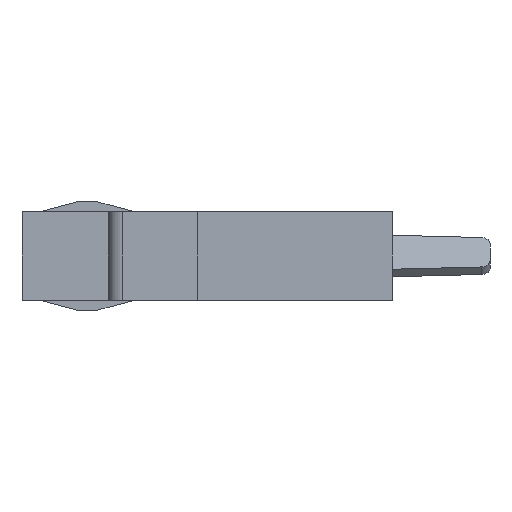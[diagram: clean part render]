
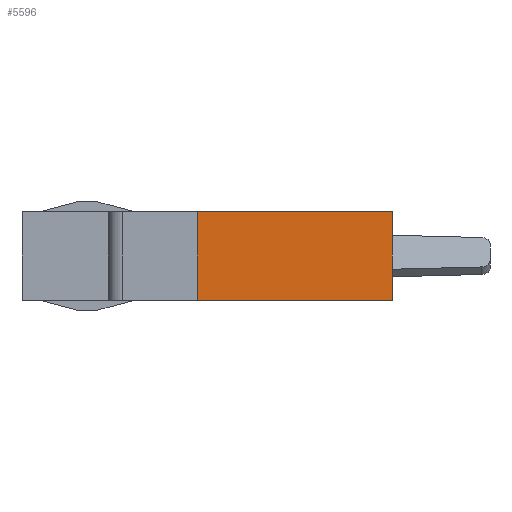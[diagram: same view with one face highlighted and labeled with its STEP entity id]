
A CAD part, left-side view. The second image highlights one B-rep face of the part: STEP entity #5596.
In plain terms, the highlighted planar face has unit normal (-1, 0, 0).
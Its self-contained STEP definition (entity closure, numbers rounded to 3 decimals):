
#51 = CARTESIAN_POINT ( 'NONE',  ( -2.235, 0., 2.54 ) ) ;
#229 = EDGE_CURVE ( 'NONE', #5375, #2570, #3643, .T. ) ;
#600 = CARTESIAN_POINT ( 'NONE',  ( -2.235, -11.176, -2.54 ) ) ;
#729 = LINE ( 'NONE', #5185, #3225 ) ;
#948 = CARTESIAN_POINT ( 'NONE',  ( -2.235, 0., 2.54 ) ) ;
#1081 = PLANE ( 'NONE',  #2968 ) ;
#1299 = LINE ( 'NONE', #3703, #6645 ) ;
#1427 = ORIENTED_EDGE ( 'NONE', *, *, #5101, .F. ) ;
#1739 = EDGE_CURVE ( 'NONE', #3036, #5375, #729, .T. ) ;
#2226 = DIRECTION ( 'NONE',  ( 0., 1., 0. ) ) ;
#2310 = LINE ( 'NONE', #948, #5884 ) ;
#2388 = DIRECTION ( 'NONE',  ( 0., 1., 0. ) ) ;
#2570 = VERTEX_POINT ( 'NONE', #51 ) ;
#2621 = DIRECTION ( 'NONE',  ( 0., 0., 1. ) ) ;
#2668 = DIRECTION ( 'NONE',  ( -1., 0., 0. ) ) ;
#2684 = ORIENTED_EDGE ( 'NONE', *, *, #1739, .T. ) ;
#2890 = CARTESIAN_POINT ( 'NONE',  ( -2.235, -11.176, 2.54 ) ) ;
#2968 = AXIS2_PLACEMENT_3D ( 'NONE', #600, #2668, #2621 ) ;
#3036 = VERTEX_POINT ( 'NONE', #5027 ) ;
#3225 = VECTOR ( 'NONE', #5701, 1000. ) ;
#3454 = VERTEX_POINT ( 'NONE', #4901 ) ;
#3611 = FACE_OUTER_BOUND ( 'NONE', #5616, .T. ) ;
#3643 = LINE ( 'NONE', #2890, #6347 ) ;
#3703 = CARTESIAN_POINT ( 'NONE',  ( -2.235, -11.176, -2.54 ) ) ;
#4626 = ORIENTED_EDGE ( 'NONE', *, *, #6004, .T. ) ;
#4901 = CARTESIAN_POINT ( 'NONE',  ( -2.235, 0., -2.54 ) ) ;
#4905 = ORIENTED_EDGE ( 'NONE', *, *, #229, .T. ) ;
#4911 = CARTESIAN_POINT ( 'NONE',  ( -2.235, -11.176, 2.54 ) ) ;
#5027 = CARTESIAN_POINT ( 'NONE',  ( -2.235, -11.176, -2.54 ) ) ;
#5101 = EDGE_CURVE ( 'NONE', #3036, #3454, #1299, .T. ) ;
#5185 = CARTESIAN_POINT ( 'NONE',  ( -2.235, -11.176, -2.54 ) ) ;
#5375 = VERTEX_POINT ( 'NONE', #4911 ) ;
#5589 = DIRECTION ( 'NONE',  ( 0., 0., -1. ) ) ;
#5596 = ADVANCED_FACE ( 'NONE', ( #3611 ), #1081, .T. ) ;
#5616 = EDGE_LOOP ( 'NONE', ( #4905, #4626, #1427, #2684 ) ) ;
#5701 = DIRECTION ( 'NONE',  ( 0., 0., 1. ) ) ;
#5884 = VECTOR ( 'NONE', #5589, 1000. ) ;
#6004 = EDGE_CURVE ( 'NONE', #2570, #3454, #2310, .T. ) ;
#6347 = VECTOR ( 'NONE', #2388, 1000. ) ;
#6645 = VECTOR ( 'NONE', #2226, 1000. ) ;
